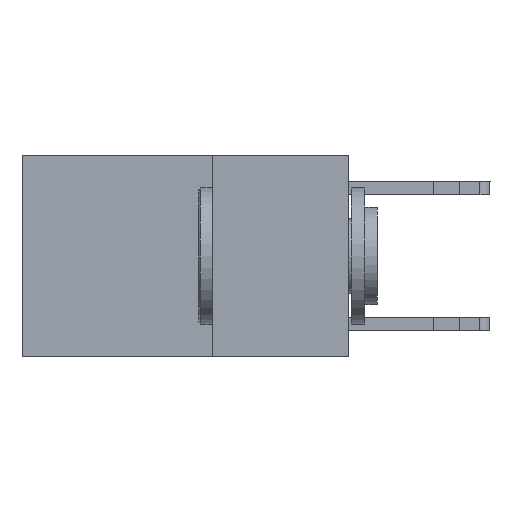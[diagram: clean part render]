
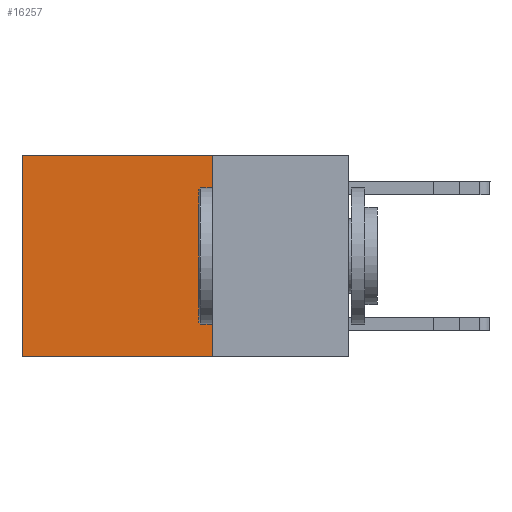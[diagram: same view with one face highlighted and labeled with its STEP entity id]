
A CAD part, left-side view. The second image highlights one B-rep face of the part: STEP entity #16257.
In plain terms, the highlighted planar face has unit normal (-1, 0, 0).
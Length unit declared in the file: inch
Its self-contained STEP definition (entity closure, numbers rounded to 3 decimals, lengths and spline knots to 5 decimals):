
#88 = CARTESIAN_POINT ( 'NONE',  ( 0.2625, 0.25, 0. ) ) ;
#831 = EDGE_LOOP ( 'NONE', ( #10822, #20755, #19552, #7506 ) ) ;
#978 = EDGE_CURVE ( 'NONE', #6512, #21851, #15208, .T. ) ;
#1793 = PLANE ( 'NONE',  #21251 ) ;
#2486 = CARTESIAN_POINT ( 'NONE',  ( 0.2625, 0.25, -0.37 ) ) ;
#3026 = LINE ( 'NONE', #19598, #12098 ) ;
#4060 = VERTEX_POINT ( 'NONE', #2486 ) ;
#5346 = VECTOR ( 'NONE', #23213, 39.37008 ) ;
#6033 = DIRECTION ( 'NONE',  ( 0., 0., -1. ) ) ;
#6417 = VERTEX_POINT ( 'NONE', #19489 ) ;
#6512 = VERTEX_POINT ( 'NONE', #18625 ) ;
#7506 = ORIENTED_EDGE ( 'NONE', *, *, #9727, .T. ) ;
#8063 = CARTESIAN_POINT ( 'NONE',  ( 0.2625, 0.25, -0.37 ) ) ;
#9506 = VECTOR ( 'NONE', #19320, 39.37008 ) ;
#9727 = EDGE_CURVE ( 'NONE', #6417, #6512, #3026, .T. ) ;
#10358 = DIRECTION ( 'NONE',  ( 0., 1., 0. ) ) ;
#10822 = ORIENTED_EDGE ( 'NONE', *, *, #978, .T. ) ;
#11762 = VECTOR ( 'NONE', #6033, 39.37008 ) ;
#12098 = VECTOR ( 'NONE', #10358, 39.37008 ) ;
#12887 = DIRECTION ( 'NONE',  ( 0., 0., -1. ) ) ;
#13858 = LINE ( 'NONE', #8063, #9506 ) ;
#14019 = CARTESIAN_POINT ( 'NONE',  ( 0.2625, 0.25, 0. ) ) ;
#14701 = FACE_OUTER_BOUND ( 'NONE', #831, .T. ) ;
#14821 = EDGE_CURVE ( 'NONE', #4060, #21851, #13858, .T. ) ;
#15208 = LINE ( 'NONE', #22495, #11762 ) ;
#15397 = DIRECTION ( 'NONE',  ( 1., 0., 0. ) ) ;
#16257 = ADVANCED_FACE ( 'NONE', ( #14701 ), #1793, .F. ) ;
#17704 = LINE ( 'NONE', #14019, #5346 ) ;
#17859 = CARTESIAN_POINT ( 'NONE',  ( 0.2625, 0.6, -0.37 ) ) ;
#18625 = CARTESIAN_POINT ( 'NONE',  ( 0.2625, 0.6, 0. ) ) ;
#18663 = EDGE_CURVE ( 'NONE', #6417, #4060, #17704, .T. ) ;
#19320 = DIRECTION ( 'NONE',  ( 0., 1., 0. ) ) ;
#19489 = CARTESIAN_POINT ( 'NONE',  ( 0.2625, 0.25, 0. ) ) ;
#19552 = ORIENTED_EDGE ( 'NONE', *, *, #18663, .F. ) ;
#19598 = CARTESIAN_POINT ( 'NONE',  ( 0.2625, 0.25, 0. ) ) ;
#20755 = ORIENTED_EDGE ( 'NONE', *, *, #14821, .F. ) ;
#21251 = AXIS2_PLACEMENT_3D ( 'NONE', #88, #15397, #12887 ) ;
#21851 = VERTEX_POINT ( 'NONE', #17859 ) ;
#22495 = CARTESIAN_POINT ( 'NONE',  ( 0.2625, 0.6, 0. ) ) ;
#23213 = DIRECTION ( 'NONE',  ( 0., 0., -1. ) ) ;
